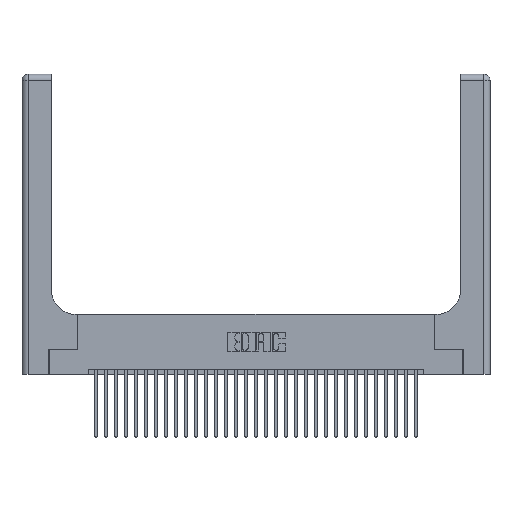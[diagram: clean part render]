
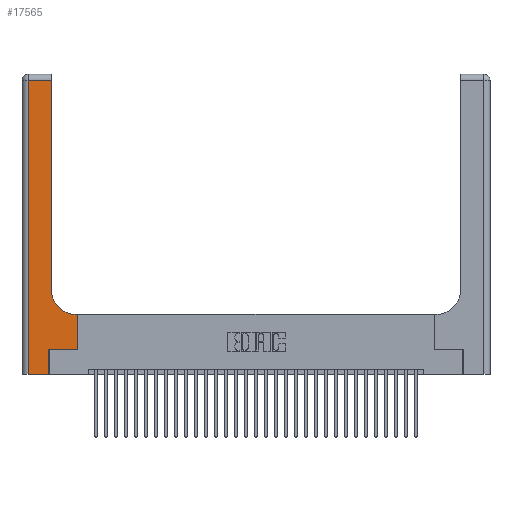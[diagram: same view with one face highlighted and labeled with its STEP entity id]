
A CAD part, top view. The second image highlights one B-rep face of the part: STEP entity #17565.
In plain terms, the highlighted planar face has unit normal (0, 0, 1).
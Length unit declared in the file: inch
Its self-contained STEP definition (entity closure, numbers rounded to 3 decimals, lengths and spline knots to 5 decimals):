
#91 = AXIS2_PLACEMENT_3D ( 'NONE', #1944, #24658, #9688 ) ;
#200 = EDGE_LOOP ( 'NONE', ( #32147, #3784, #3560, #19431, #28639, #19677, #2844, #24808, #27718 ) ) ;
#1045 = PLANE ( 'NONE',  #11249 ) ;
#1078 = LINE ( 'NONE', #25725, #12813 ) ;
#1452 = VERTEX_POINT ( 'NONE', #23821 ) ;
#1944 = CARTESIAN_POINT ( 'NONE',  ( 0.5415, 0.85, 0.37 ) ) ;
#2432 = LINE ( 'NONE', #22302, #15701 ) ;
#2844 = ORIENTED_EDGE ( 'NONE', *, *, #21381, .T. ) ;
#3240 = VERTEX_POINT ( 'NONE', #26501 ) ;
#3560 = ORIENTED_EDGE ( 'NONE', *, *, #30460, .T. ) ;
#3784 = ORIENTED_EDGE ( 'NONE', *, *, #13458, .T. ) ;
#3863 = DIRECTION ( 'NONE',  ( 0., 1., 0. ) ) ;
#3972 = CARTESIAN_POINT ( 'NONE',  ( 0.5415, 0.6, 0.37 ) ) ;
#4067 = VECTOR ( 'NONE', #6993, 39.37008 ) ;
#5180 = VECTOR ( 'NONE', #13977, 39.37008 ) ;
#5575 = VECTOR ( 'NONE', #9000, 39.37008 ) ;
#5946 = LINE ( 'NONE', #21149, #5180 ) ;
#6754 = EDGE_CURVE ( 'NONE', #18192, #1452, #10178, .T. ) ;
#6993 = DIRECTION ( 'NONE',  ( 0., 1., 0. ) ) ;
#8204 = VERTEX_POINT ( 'NONE', #20418 ) ;
#8312 = CARTESIAN_POINT ( 'NONE',  ( 0., 0., 0.37 ) ) ;
#8678 = DIRECTION ( 'NONE',  ( -1., 0., 0. ) ) ;
#9000 = DIRECTION ( 'NONE',  ( -1., 0., 0. ) ) ;
#9688 = DIRECTION ( 'NONE',  ( 1., 0., 0. ) ) ;
#10178 = LINE ( 'NONE', #8312, #14879 ) ;
#10700 = LINE ( 'NONE', #24703, #4067 ) ;
#10995 = EDGE_CURVE ( 'NONE', #13470, #8204, #23722, .T. ) ;
#11151 = VERTEX_POINT ( 'NONE', #22440 ) ;
#11249 = AXIS2_PLACEMENT_3D ( 'NONE', #23626, #26247, #8678 ) ;
#11295 = DIRECTION ( 'NONE',  ( 0., -1., 0. ) ) ;
#12813 = VECTOR ( 'NONE', #15809, 39.37008 ) ;
#13458 = EDGE_CURVE ( 'NONE', #31741, #17338, #26298, .T. ) ;
#13470 = VERTEX_POINT ( 'NONE', #3972 ) ;
#13596 = VECTOR ( 'NONE', #11295, 39.37008 ) ;
#13745 = FACE_OUTER_BOUND ( 'NONE', #200, .T. ) ;
#13823 = EDGE_CURVE ( 'NONE', #1452, #11151, #5946, .T. ) ;
#13977 = DIRECTION ( 'NONE',  ( 0., 1., 0. ) ) ;
#14629 = EDGE_CURVE ( 'NONE', #11151, #20945, #2432, .T. ) ;
#14702 = DIRECTION ( 'NONE',  ( 1., 0., 0. ) ) ;
#14879 = VECTOR ( 'NONE', #15863, 39.37008 ) ;
#14955 = CARTESIAN_POINT ( 'NONE',  ( 0.5585, 0.25, 0.37 ) ) ;
#15701 = VECTOR ( 'NONE', #14702, 39.37008 ) ;
#15809 = DIRECTION ( 'NONE',  ( -1., 0., 0. ) ) ;
#15863 = DIRECTION ( 'NONE',  ( 1., 0., 0. ) ) ;
#17338 = VERTEX_POINT ( 'NONE', #27803 ) ;
#17565 = ADVANCED_FACE ( 'NONE', ( #13745 ), #1045, .F. ) ;
#18192 = VERTEX_POINT ( 'NONE', #28841 ) ;
#18284 = CARTESIAN_POINT ( 'NONE',  ( 0.06, 3., 0.37 ) ) ;
#18627 = LINE ( 'NONE', #18284, #13596 ) ;
#19056 = CARTESIAN_POINT ( 'NONE',  ( 0.5585, 0.25, 0.37 ) ) ;
#19431 = ORIENTED_EDGE ( 'NONE', *, *, #6754, .T. ) ;
#19553 = LINE ( 'NONE', #19056, #24235 ) ;
#19677 = ORIENTED_EDGE ( 'NONE', *, *, #14629, .T. ) ;
#20418 = CARTESIAN_POINT ( 'NONE',  ( 0.2915, 0.85, 0.37 ) ) ;
#20945 = VERTEX_POINT ( 'NONE', #14955 ) ;
#21149 = CARTESIAN_POINT ( 'NONE',  ( 0.269, 0., 0.37 ) ) ;
#21381 = EDGE_CURVE ( 'NONE', #20945, #3240, #19553, .T. ) ;
#22302 = CARTESIAN_POINT ( 'NONE',  ( 0.269, 0.25, 0.37 ) ) ;
#22440 = CARTESIAN_POINT ( 'NONE',  ( 0.269, 0.25, 0.37 ) ) ;
#23626 = CARTESIAN_POINT ( 'NONE',  ( 0., 3., 0.37 ) ) ;
#23722 = CIRCLE ( 'NONE', #91, 0.25 ) ;
#23821 = CARTESIAN_POINT ( 'NONE',  ( 0.269, 0., 0.37 ) ) ;
#24235 = VECTOR ( 'NONE', #3863, 39.37008 ) ;
#24658 = DIRECTION ( 'NONE',  ( 0., 0., -1. ) ) ;
#24703 = CARTESIAN_POINT ( 'NONE',  ( 0.2915, 3., 0.37 ) ) ;
#24808 = ORIENTED_EDGE ( 'NONE', *, *, #30399, .T. ) ;
#25725 = CARTESIAN_POINT ( 'NONE',  ( 0.2915, 0.6, 0.37 ) ) ;
#25747 = EDGE_CURVE ( 'NONE', #8204, #31741, #10700, .T. ) ;
#26247 = DIRECTION ( 'NONE',  ( 0., 0., -1. ) ) ;
#26298 = LINE ( 'NONE', #29213, #5575 ) ;
#26501 = CARTESIAN_POINT ( 'NONE',  ( 0.5585, 0.6, 0.37 ) ) ;
#27718 = ORIENTED_EDGE ( 'NONE', *, *, #10995, .T. ) ;
#27803 = CARTESIAN_POINT ( 'NONE',  ( 0.06, 2.94, 0.37 ) ) ;
#28639 = ORIENTED_EDGE ( 'NONE', *, *, #13823, .T. ) ;
#28841 = CARTESIAN_POINT ( 'NONE',  ( 0.06, 0., 0.37 ) ) ;
#29213 = CARTESIAN_POINT ( 'NONE',  ( 0., 2.94, 0.37 ) ) ;
#30215 = CARTESIAN_POINT ( 'NONE',  ( 0.2915, 2.94, 0.37 ) ) ;
#30399 = EDGE_CURVE ( 'NONE', #3240, #13470, #1078, .T. ) ;
#30460 = EDGE_CURVE ( 'NONE', #17338, #18192, #18627, .T. ) ;
#31741 = VERTEX_POINT ( 'NONE', #30215 ) ;
#32147 = ORIENTED_EDGE ( 'NONE', *, *, #25747, .T. ) ;
